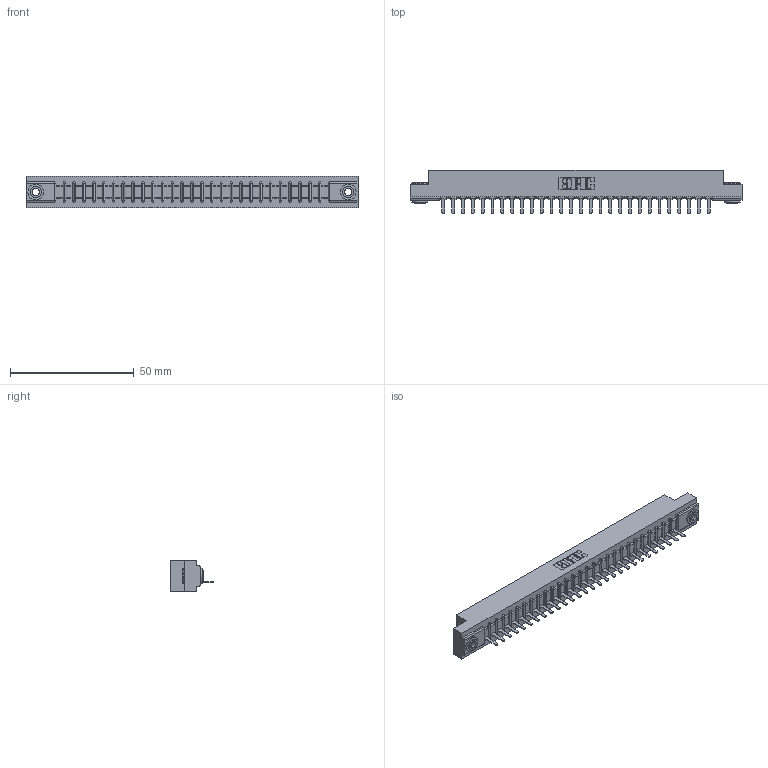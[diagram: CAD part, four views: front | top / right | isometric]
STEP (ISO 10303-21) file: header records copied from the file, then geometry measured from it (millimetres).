
FILE_DESCRIPTION (( 'STEP AP203' ), '1' );
FILE_NAME ('357-028-421-103.STEP', '2020-10-01T21:35:55', ( '' ), ( '' ), 'SwSTEP 2.0', 'SolidWorks 2020', '' );
FILE_SCHEMA (( 'CONFIG_CONTROL_DESIGN' ));
Length unit declared in the file: inch
Products named in the file (4): 345-250-002_345-250-002-102; 357-028-421-103; 307 Part_.156 Dia Mounting Holes; 307-290-002_521
Assembly tree (31 placements, depth 2):
  357-028-421-103
    307 Part_.156 Dia Mounting Holes
    307-290-002_521  x28
    345-250-002_345-250-002-102  x2
Bounding box: 133.96 x 17.42 x 12.7 mm (x, y, z)
Volume: 14233.9 mm3; surface area: 17844.6 mm2
Topology: 31 solids, 31 shells, 2271 faces, 6931 edges, 4538 vertices
Faces by surface type: plane 1354, cylinder 851, sphere 58, cone 8
Entity records: 27513 total; most frequent: CARTESIAN_POINT 4617, ORIENTED_EDGE 4598, DIRECTION 4507, EDGE_CURVE 2299, VECTOR 1747, LINE 1747, VERTEX_POINT 1490, AXIS2_PLACEMENT_3D 1380
